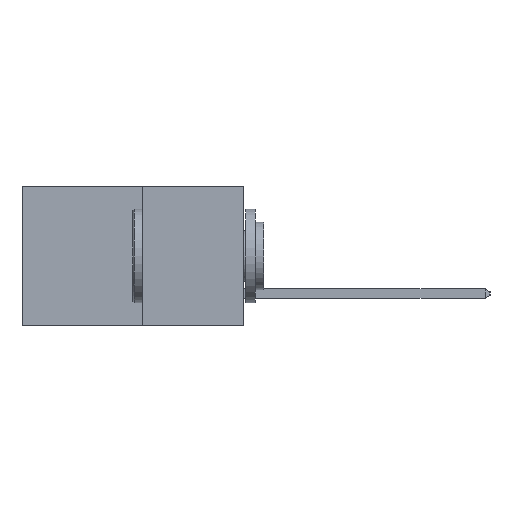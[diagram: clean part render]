
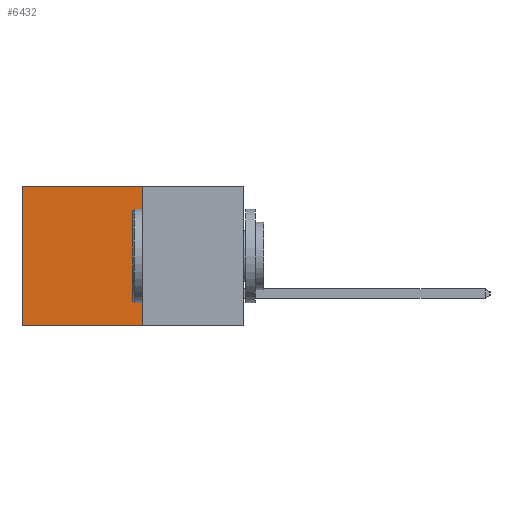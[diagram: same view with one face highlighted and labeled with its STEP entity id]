
A CAD part, left-side view. The second image highlights one B-rep face of the part: STEP entity #6432.
In plain terms, the highlighted planar face has unit normal (-1, 0, 0).
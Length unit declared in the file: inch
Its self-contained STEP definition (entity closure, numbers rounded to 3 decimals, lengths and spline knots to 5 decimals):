
#34 = LINE ( 'NONE', #1327, #4021 ) ;
#1011 = DIRECTION ( 'NONE',  ( 0., 0., -1. ) ) ;
#1323 = CARTESIAN_POINT ( 'NONE',  ( 0.277, 0.27, -0.37 ) ) ;
#1327 = CARTESIAN_POINT ( 'NONE',  ( 0.277, 0.27, 0. ) ) ;
#1440 = VERTEX_POINT ( 'NONE', #4276 ) ;
#1489 = DIRECTION ( 'NONE',  ( 0., 0., -1. ) ) ;
#1517 = ORIENTED_EDGE ( 'NONE', *, *, #2683, .T. ) ;
#1646 = CARTESIAN_POINT ( 'NONE',  ( 0.277, 0.27, -0.37 ) ) ;
#2129 = VERTEX_POINT ( 'NONE', #1323 ) ;
#2430 = ORIENTED_EDGE ( 'NONE', *, *, #4223, .F. ) ;
#2683 = EDGE_CURVE ( 'NONE', #9413, #10551, #34, .T. ) ;
#3243 = PLANE ( 'NONE',  #7806 ) ;
#4021 = VECTOR ( 'NONE', #6709, 39.37008 ) ;
#4069 = DIRECTION ( 'NONE',  ( 0., 0., -1. ) ) ;
#4223 = EDGE_CURVE ( 'NONE', #9413, #2129, #9008, .T. ) ;
#4276 = CARTESIAN_POINT ( 'NONE',  ( 0.277, 0.59, -0.37 ) ) ;
#4356 = EDGE_CURVE ( 'NONE', #2129, #1440, #9659, .T. ) ;
#4404 = CARTESIAN_POINT ( 'NONE',  ( 0.277, 0.59, -0.37 ) ) ;
#5398 = EDGE_LOOP ( 'NONE', ( #7631, #8514, #2430, #1517 ) ) ;
#5492 = FACE_OUTER_BOUND ( 'NONE', #5398, .T. ) ;
#5736 = LINE ( 'NONE', #4404, #9849 ) ;
#6432 = ADVANCED_FACE ( 'NONE', ( #5492 ), #3243, .F. ) ;
#6542 = CARTESIAN_POINT ( 'NONE',  ( 0.277, 0.27, -0.37 ) ) ;
#6586 = VECTOR ( 'NONE', #1489, 39.37008 ) ;
#6709 = DIRECTION ( 'NONE',  ( 0., 1., 0. ) ) ;
#6901 = CARTESIAN_POINT ( 'NONE',  ( 0.277, 0.27, 0. ) ) ;
#7453 = CARTESIAN_POINT ( 'NONE',  ( 0.277, 0.59, 0. ) ) ;
#7485 = VECTOR ( 'NONE', #9113, 39.37008 ) ;
#7631 = ORIENTED_EDGE ( 'NONE', *, *, #10716, .T. ) ;
#7806 = AXIS2_PLACEMENT_3D ( 'NONE', #6542, #8998, #4069 ) ;
#8514 = ORIENTED_EDGE ( 'NONE', *, *, #4356, .F. ) ;
#8998 = DIRECTION ( 'NONE',  ( 1., 0., 0. ) ) ;
#9008 = LINE ( 'NONE', #1646, #6586 ) ;
#9113 = DIRECTION ( 'NONE',  ( 0., 1., 0. ) ) ;
#9413 = VERTEX_POINT ( 'NONE', #6901 ) ;
#9659 = LINE ( 'NONE', #10169, #7485 ) ;
#9849 = VECTOR ( 'NONE', #1011, 39.37008 ) ;
#10169 = CARTESIAN_POINT ( 'NONE',  ( 0.277, 0.27, -0.37 ) ) ;
#10551 = VERTEX_POINT ( 'NONE', #7453 ) ;
#10716 = EDGE_CURVE ( 'NONE', #10551, #1440, #5736, .T. ) ;
